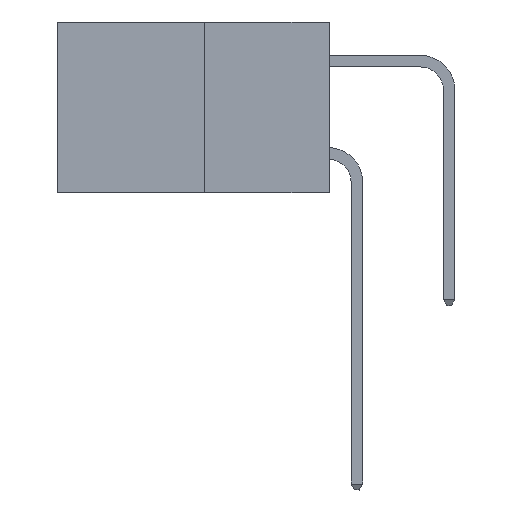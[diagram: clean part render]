
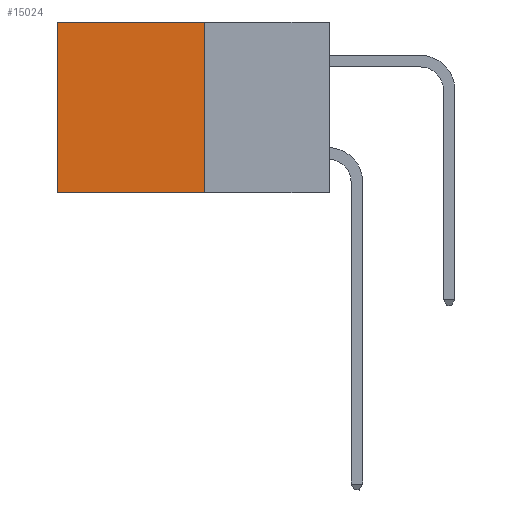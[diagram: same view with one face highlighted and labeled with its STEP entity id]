
A CAD part, left-side view. The second image highlights one B-rep face of the part: STEP entity #15024.
In plain terms, the highlighted planar face has unit normal (-1, 0, 0).
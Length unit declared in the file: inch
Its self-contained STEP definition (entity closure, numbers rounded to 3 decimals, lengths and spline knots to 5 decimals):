
#27 = VERTEX_POINT ( 'NONE', #110 ) ;
#110 = CARTESIAN_POINT ( 'NONE',  ( 0.277, 0.59, -0.37 ) ) ;
#1986 = CARTESIAN_POINT ( 'NONE',  ( 0.277, 0.27, -0.37 ) ) ;
#3084 = ORIENTED_EDGE ( 'NONE', *, *, #17227, .F. ) ;
#3158 = EDGE_CURVE ( 'NONE', #13853, #14119, #14381, .T. ) ;
#3575 = VECTOR ( 'NONE', #4253, 39.37008 ) ;
#3642 = DIRECTION ( 'NONE',  ( 0., 0., -1. ) ) ;
#4253 = DIRECTION ( 'NONE',  ( 0., 0., -1. ) ) ;
#4453 = DIRECTION ( 'NONE',  ( 0., 1., 0. ) ) ;
#4510 = ORIENTED_EDGE ( 'NONE', *, *, #18387, .F. ) ;
#5234 = PLANE ( 'NONE',  #8115 ) ;
#7260 = VECTOR ( 'NONE', #9338, 39.37008 ) ;
#7717 = LINE ( 'NONE', #16863, #15361 ) ;
#8115 = AXIS2_PLACEMENT_3D ( 'NONE', #1986, #13485, #3642 ) ;
#8780 = DIRECTION ( 'NONE',  ( 0., 1., 0. ) ) ;
#9338 = DIRECTION ( 'NONE',  ( 0., 0., -1. ) ) ;
#10091 = VECTOR ( 'NONE', #4453, 39.37008 ) ;
#11130 = ORIENTED_EDGE ( 'NONE', *, *, #3158, .T. ) ;
#12328 = EDGE_CURVE ( 'NONE', #14119, #27, #20899, .T. ) ;
#13485 = DIRECTION ( 'NONE',  ( 1., 0., 0. ) ) ;
#13853 = VERTEX_POINT ( 'NONE', #17004 ) ;
#14119 = VERTEX_POINT ( 'NONE', #17667 ) ;
#14381 = LINE ( 'NONE', #17332, #10091 ) ;
#14555 = CARTESIAN_POINT ( 'NONE',  ( 0.277, 0.27, -0.37 ) ) ;
#14595 = ORIENTED_EDGE ( 'NONE', *, *, #12328, .T. ) ;
#15024 = ADVANCED_FACE ( 'NONE', ( #16823 ), #5234, .F. ) ;
#15045 = EDGE_LOOP ( 'NONE', ( #14595, #4510, #3084, #11130 ) ) ;
#15361 = VECTOR ( 'NONE', #8780, 39.37008 ) ;
#16823 = FACE_OUTER_BOUND ( 'NONE', #15045, .T. ) ;
#16863 = CARTESIAN_POINT ( 'NONE',  ( 0.277, 0.27, -0.37 ) ) ;
#17004 = CARTESIAN_POINT ( 'NONE',  ( 0.277, 0.27, 0. ) ) ;
#17227 = EDGE_CURVE ( 'NONE', #13853, #17407, #20228, .T. ) ;
#17332 = CARTESIAN_POINT ( 'NONE',  ( 0.277, 0.27, 0. ) ) ;
#17407 = VERTEX_POINT ( 'NONE', #14555 ) ;
#17667 = CARTESIAN_POINT ( 'NONE',  ( 0.277, 0.59, 0. ) ) ;
#18387 = EDGE_CURVE ( 'NONE', #17407, #27, #7717, .T. ) ;
#18990 = CARTESIAN_POINT ( 'NONE',  ( 0.277, 0.27, -0.37 ) ) ;
#20228 = LINE ( 'NONE', #18990, #7260 ) ;
#20479 = CARTESIAN_POINT ( 'NONE',  ( 0.277, 0.59, -0.37 ) ) ;
#20899 = LINE ( 'NONE', #20479, #3575 ) ;
